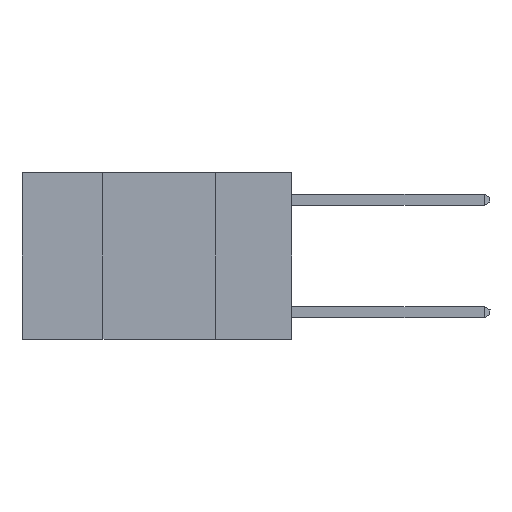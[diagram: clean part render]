
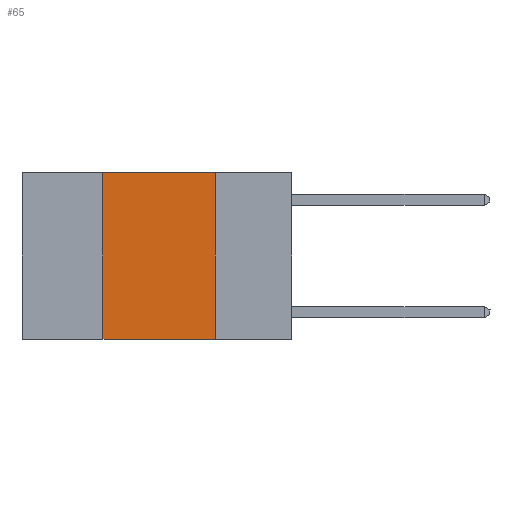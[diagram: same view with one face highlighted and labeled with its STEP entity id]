
A CAD part, left-side view. The second image highlights one B-rep face of the part: STEP entity #65.
In plain terms, the highlighted planar face has unit normal (-1, 0, 0).
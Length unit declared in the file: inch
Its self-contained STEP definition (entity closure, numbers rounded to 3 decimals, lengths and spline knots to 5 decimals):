
#65 = ADVANCED_FACE ( 'NONE', ( #879 ), #6169, .F. ) ;
#408 = CARTESIAN_POINT ( 'NONE',  ( 0., 0.6, -0.37 ) ) ;
#452 = ORIENTED_EDGE ( 'NONE', *, *, #6727, .F. ) ;
#879 = FACE_OUTER_BOUND ( 'NONE', #2666, .T. ) ;
#1081 = DIRECTION ( 'NONE',  ( 0., -1., 0. ) ) ;
#1188 = DIRECTION ( 'NONE',  ( 0., -1., 0. ) ) ;
#1245 = CARTESIAN_POINT ( 'NONE',  ( 0., 0.42, 0. ) ) ;
#1489 = CARTESIAN_POINT ( 'NONE',  ( 0., 0.6, 0. ) ) ;
#1804 = VERTEX_POINT ( 'NONE', #1245 ) ;
#1825 = VECTOR ( 'NONE', #1188, 39.37008 ) ;
#2167 = LINE ( 'NONE', #8803, #5927 ) ;
#2238 = ORIENTED_EDGE ( 'NONE', *, *, #9396, .T. ) ;
#2666 = EDGE_LOOP ( 'NONE', ( #8447, #452, #6677, #2238 ) ) ;
#3756 = VECTOR ( 'NONE', #5254, 39.37008 ) ;
#3919 = LINE ( 'NONE', #408, #1825 ) ;
#4438 = CARTESIAN_POINT ( 'NONE',  ( 0., 0.42, -0.37 ) ) ;
#5254 = DIRECTION ( 'NONE',  ( 0., 0., 1. ) ) ;
#5395 = DIRECTION ( 'NONE',  ( 0., 0., -1. ) ) ;
#5668 = LINE ( 'NONE', #5946, #3756 ) ;
#5927 = VECTOR ( 'NONE', #6706, 39.37008 ) ;
#5946 = CARTESIAN_POINT ( 'NONE',  ( 0., 0.42, 0. ) ) ;
#6079 = VERTEX_POINT ( 'NONE', #4438 ) ;
#6160 = DIRECTION ( 'NONE',  ( 1., 0., 0. ) ) ;
#6169 = PLANE ( 'NONE',  #7733 ) ;
#6677 = ORIENTED_EDGE ( 'NONE', *, *, #6924, .F. ) ;
#6706 = DIRECTION ( 'NONE',  ( 0., 0., -1. ) ) ;
#6727 = EDGE_CURVE ( 'NONE', #1804, #7770, #7816, .T. ) ;
#6924 = EDGE_CURVE ( 'NONE', #6079, #1804, #5668, .T. ) ;
#7085 = CARTESIAN_POINT ( 'NONE',  ( 0., 0.17, -0.37 ) ) ;
#7733 = AXIS2_PLACEMENT_3D ( 'NONE', #1489, #6160, #5395 ) ;
#7770 = VERTEX_POINT ( 'NONE', #8641 ) ;
#7816 = LINE ( 'NONE', #8328, #9397 ) ;
#8328 = CARTESIAN_POINT ( 'NONE',  ( 0., 0.6, 0. ) ) ;
#8378 = VERTEX_POINT ( 'NONE', #7085 ) ;
#8447 = ORIENTED_EDGE ( 'NONE', *, *, #8908, .F. ) ;
#8641 = CARTESIAN_POINT ( 'NONE',  ( 0., 0.17, 0. ) ) ;
#8803 = CARTESIAN_POINT ( 'NONE',  ( 0., 0.17, 0. ) ) ;
#8908 = EDGE_CURVE ( 'NONE', #7770, #8378, #2167, .T. ) ;
#9396 = EDGE_CURVE ( 'NONE', #6079, #8378, #3919, .T. ) ;
#9397 = VECTOR ( 'NONE', #1081, 39.37008 ) ;
